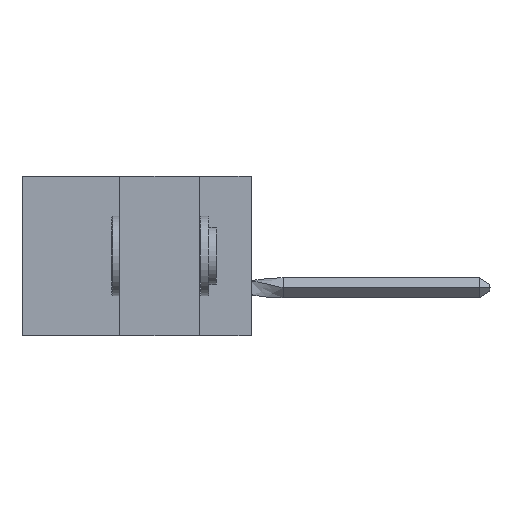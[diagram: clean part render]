
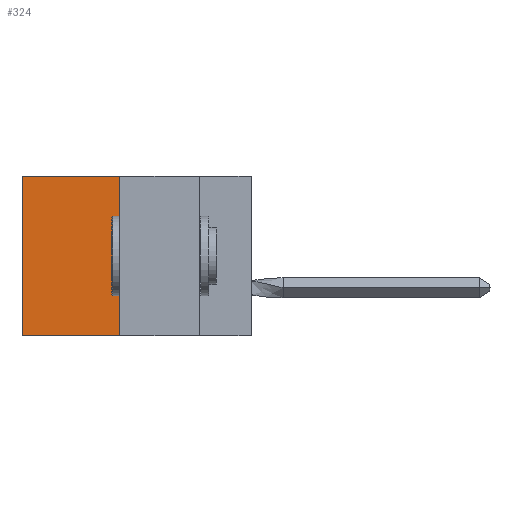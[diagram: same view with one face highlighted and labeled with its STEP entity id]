
A CAD part, left-side view. The second image highlights one B-rep face of the part: STEP entity #324.
In plain terms, the highlighted planar face has unit normal (-1, 0, 0).
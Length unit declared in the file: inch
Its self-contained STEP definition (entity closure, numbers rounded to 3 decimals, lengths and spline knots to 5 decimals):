
#324 = ADVANCED_FACE ( 'NONE', ( #2390 ), #10553, .F. ) ;
#1134 = EDGE_CURVE ( 'NONE', #9305, #15337, #13526, .T. ) ;
#1163 = VECTOR ( 'NONE', #12327, 39.37008 ) ;
#2069 = DIRECTION ( 'NONE',  ( 0., 0., -1. ) ) ;
#2390 = FACE_OUTER_BOUND ( 'NONE', #5839, .T. ) ;
#2391 = CARTESIAN_POINT ( 'NONE',  ( 0.305, 0.72, 0. ) ) ;
#2424 = ORIENTED_EDGE ( 'NONE', *, *, #1134, .F. ) ;
#3247 = DIRECTION ( 'NONE',  ( 1., 0., 0. ) ) ;
#3814 = CARTESIAN_POINT ( 'NONE',  ( 0.305, 0.413, -0.5 ) ) ;
#3989 = VECTOR ( 'NONE', #13840, 39.37008 ) ;
#4029 = VECTOR ( 'NONE', #2069, 39.37008 ) ;
#5204 = CARTESIAN_POINT ( 'NONE',  ( 0.305, 0.72, -0.5 ) ) ;
#5839 = EDGE_LOOP ( 'NONE', ( #6265, #9652, #2424, #12901 ) ) ;
#6265 = ORIENTED_EDGE ( 'NONE', *, *, #9201, .T. ) ;
#6280 = CARTESIAN_POINT ( 'NONE',  ( 0.305, 0.413, 0. ) ) ;
#6321 = DIRECTION ( 'NONE',  ( 0., 1., 0. ) ) ;
#6768 = CARTESIAN_POINT ( 'NONE',  ( 0.305, 0.413, -0.5 ) ) ;
#6908 = LINE ( 'NONE', #7108, #4029 ) ;
#6916 = CARTESIAN_POINT ( 'NONE',  ( 0.305, 0.413, -0.5 ) ) ;
#7108 = CARTESIAN_POINT ( 'NONE',  ( 0.305, 0.72, -0.5 ) ) ;
#8301 = LINE ( 'NONE', #6280, #13578 ) ;
#9201 = EDGE_CURVE ( 'NONE', #9521, #10590, #6908, .T. ) ;
#9305 = VERTEX_POINT ( 'NONE', #9458 ) ;
#9458 = CARTESIAN_POINT ( 'NONE',  ( 0.305, 0.413, 0. ) ) ;
#9521 = VERTEX_POINT ( 'NONE', #2391 ) ;
#9652 = ORIENTED_EDGE ( 'NONE', *, *, #10102, .F. ) ;
#10102 = EDGE_CURVE ( 'NONE', #15337, #10590, #11434, .T. ) ;
#10371 = CARTESIAN_POINT ( 'NONE',  ( 0.305, 0.413, -0.5 ) ) ;
#10553 = PLANE ( 'NONE',  #14137 ) ;
#10590 = VERTEX_POINT ( 'NONE', #5204 ) ;
#11434 = LINE ( 'NONE', #10371, #3989 ) ;
#12327 = DIRECTION ( 'NONE',  ( 0., 0., -1. ) ) ;
#12901 = ORIENTED_EDGE ( 'NONE', *, *, #15740, .T. ) ;
#12972 = DIRECTION ( 'NONE',  ( 0., 0., -1. ) ) ;
#13526 = LINE ( 'NONE', #3814, #1163 ) ;
#13578 = VECTOR ( 'NONE', #6321, 39.37008 ) ;
#13840 = DIRECTION ( 'NONE',  ( 0., 1., 0. ) ) ;
#14137 = AXIS2_PLACEMENT_3D ( 'NONE', #6768, #3247, #12972 ) ;
#15337 = VERTEX_POINT ( 'NONE', #6916 ) ;
#15740 = EDGE_CURVE ( 'NONE', #9305, #9521, #8301, .T. ) ;
